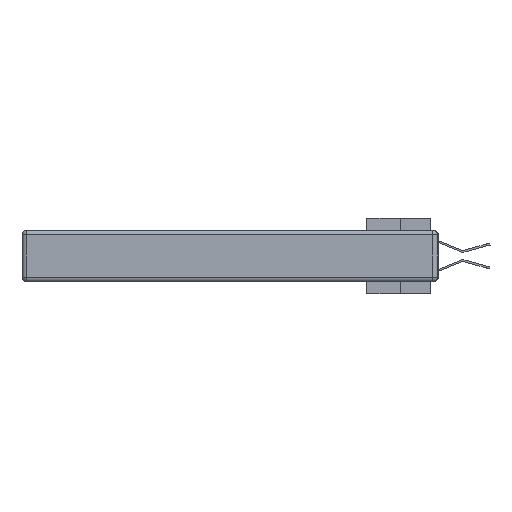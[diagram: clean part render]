
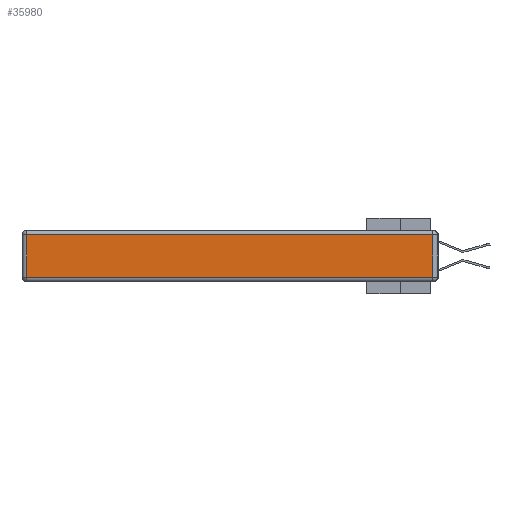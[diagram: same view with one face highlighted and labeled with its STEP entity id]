
A CAD part, left-side view. The second image highlights one B-rep face of the part: STEP entity #35980.
In plain terms, the highlighted planar face has unit normal (-1, 0, 0).
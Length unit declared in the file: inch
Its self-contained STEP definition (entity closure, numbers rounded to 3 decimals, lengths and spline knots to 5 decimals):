
#240 = EDGE_LOOP ( 'NONE', ( #22650, #35596, #14642, #30916 ) ) ;
#560 = VECTOR ( 'NONE', #25259, 39.37008 ) ;
#834 = DIRECTION ( 'NONE',  ( 0., 0., -1. ) ) ;
#1280 = CARTESIAN_POINT ( 'NONE',  ( 0., 0.03, -0.313 ) ) ;
#1888 = CARTESIAN_POINT ( 'NONE',  ( 0., 0., -0.343 ) ) ;
#2435 = VECTOR ( 'NONE', #17239, 39.37008 ) ;
#3314 = DIRECTION ( 'NONE',  ( 0., 1., 0. ) ) ;
#3574 = CARTESIAN_POINT ( 'NONE',  ( 0., 0.03, -0.343 ) ) ;
#6059 = CARTESIAN_POINT ( 'NONE',  ( 0., 0.03, -0.03 ) ) ;
#9172 = EDGE_CURVE ( 'NONE', #22452, #36787, #25327, .T. ) ;
#10148 = EDGE_CURVE ( 'NONE', #39147, #22452, #30615, .T. ) ;
#10699 = VECTOR ( 'NONE', #3314, 39.37008 ) ;
#12320 = CARTESIAN_POINT ( 'NONE',  ( 0., 2.75, -0.03 ) ) ;
#14642 = ORIENTED_EDGE ( 'NONE', *, *, #18486, .T. ) ;
#16079 = CARTESIAN_POINT ( 'NONE',  ( 0., 2.72, -0.343 ) ) ;
#17239 = DIRECTION ( 'NONE',  ( 0., -1., 0. ) ) ;
#17731 = FACE_OUTER_BOUND ( 'NONE', #240, .T. ) ;
#18486 = EDGE_CURVE ( 'NONE', #36787, #25631, #36417, .T. ) ;
#20084 = CARTESIAN_POINT ( 'NONE',  ( 0., 0., -0.313 ) ) ;
#20917 = EDGE_CURVE ( 'NONE', #25631, #39147, #24524, .T. ) ;
#20958 = AXIS2_PLACEMENT_3D ( 'NONE', #1888, #38821, #26330 ) ;
#22452 = VERTEX_POINT ( 'NONE', #1280 ) ;
#22650 = ORIENTED_EDGE ( 'NONE', *, *, #10148, .T. ) ;
#24524 = LINE ( 'NONE', #16079, #40105 ) ;
#25110 = CARTESIAN_POINT ( 'NONE',  ( 0., 2.72, -0.03 ) ) ;
#25259 = DIRECTION ( 'NONE',  ( 0., 0., 1. ) ) ;
#25327 = LINE ( 'NONE', #3574, #560 ) ;
#25631 = VERTEX_POINT ( 'NONE', #25110 ) ;
#26330 = DIRECTION ( 'NONE',  ( 0., 0., 1. ) ) ;
#30615 = LINE ( 'NONE', #20084, #2435 ) ;
#30916 = ORIENTED_EDGE ( 'NONE', *, *, #20917, .T. ) ;
#35596 = ORIENTED_EDGE ( 'NONE', *, *, #9172, .T. ) ;
#35980 = ADVANCED_FACE ( 'NONE', ( #17731 ), #39238, .T. ) ;
#36274 = CARTESIAN_POINT ( 'NONE',  ( 0., 2.72, -0.313 ) ) ;
#36417 = LINE ( 'NONE', #12320, #10699 ) ;
#36787 = VERTEX_POINT ( 'NONE', #6059 ) ;
#38821 = DIRECTION ( 'NONE',  ( -1., 0., 0. ) ) ;
#39147 = VERTEX_POINT ( 'NONE', #36274 ) ;
#39238 = PLANE ( 'NONE',  #20958 ) ;
#40105 = VECTOR ( 'NONE', #834, 39.37008 ) ;
